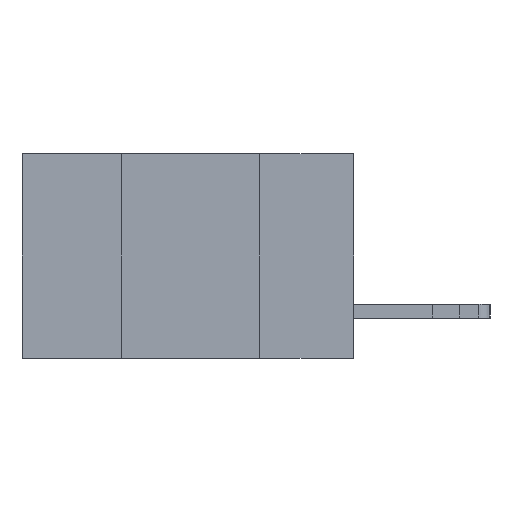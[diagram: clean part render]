
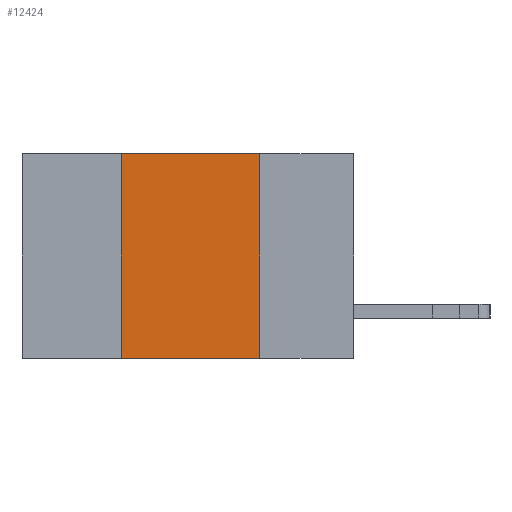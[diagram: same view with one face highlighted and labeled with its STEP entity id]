
A CAD part, left-side view. The second image highlights one B-rep face of the part: STEP entity #12424.
In plain terms, the highlighted planar face has unit normal (-1, 0, 0).
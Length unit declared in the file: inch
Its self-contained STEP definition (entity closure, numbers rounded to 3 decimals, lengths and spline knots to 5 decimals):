
#38 = ORIENTED_EDGE ( 'NONE', *, *, #11321, .T. ) ;
#1135 = PLANE ( 'NONE',  #7388 ) ;
#2249 = LINE ( 'NONE', #14327, #2546 ) ;
#2467 = VERTEX_POINT ( 'NONE', #12684 ) ;
#2546 = VECTOR ( 'NONE', #13043, 39.37008 ) ;
#2879 = DIRECTION ( 'NONE',  ( 0., 0., -1. ) ) ;
#2998 = EDGE_LOOP ( 'NONE', ( #4206, #7370, #8104, #38 ) ) ;
#3791 = CARTESIAN_POINT ( 'NONE',  ( 0., 0.17, 0. ) ) ;
#4206 = ORIENTED_EDGE ( 'NONE', *, *, #8826, .F. ) ;
#5432 = VECTOR ( 'NONE', #2879, 39.37008 ) ;
#5677 = VERTEX_POINT ( 'NONE', #6465 ) ;
#5744 = VERTEX_POINT ( 'NONE', #3791 ) ;
#6008 = CARTESIAN_POINT ( 'NONE',  ( 0., 0.6, 0. ) ) ;
#6465 = CARTESIAN_POINT ( 'NONE',  ( 0., 0.42, -0.37 ) ) ;
#7208 = VECTOR ( 'NONE', #13847, 39.37008 ) ;
#7370 = ORIENTED_EDGE ( 'NONE', *, *, #10621, .F. ) ;
#7388 = AXIS2_PLACEMENT_3D ( 'NONE', #16301, #15054, #8545 ) ;
#7578 = FACE_OUTER_BOUND ( 'NONE', #2998, .T. ) ;
#8104 = ORIENTED_EDGE ( 'NONE', *, *, #16740, .F. ) ;
#8545 = DIRECTION ( 'NONE',  ( 0., 0., -1. ) ) ;
#8826 = EDGE_CURVE ( 'NONE', #5744, #14418, #10849, .T. ) ;
#10621 = EDGE_CURVE ( 'NONE', #2467, #5744, #14060, .T. ) ;
#10849 = LINE ( 'NONE', #16007, #5432 ) ;
#11321 = EDGE_CURVE ( 'NONE', #5677, #14418, #12236, .T. ) ;
#12236 = LINE ( 'NONE', #12313, #7208 ) ;
#12313 = CARTESIAN_POINT ( 'NONE',  ( 0., 0.6, -0.37 ) ) ;
#12424 = ADVANCED_FACE ( 'NONE', ( #7578 ), #1135, .F. ) ;
#12659 = CARTESIAN_POINT ( 'NONE',  ( 0., 0.17, -0.37 ) ) ;
#12684 = CARTESIAN_POINT ( 'NONE',  ( 0., 0.42, 0. ) ) ;
#13043 = DIRECTION ( 'NONE',  ( 0., 0., 1. ) ) ;
#13847 = DIRECTION ( 'NONE',  ( 0., -1., 0. ) ) ;
#14060 = LINE ( 'NONE', #6008, #15450 ) ;
#14327 = CARTESIAN_POINT ( 'NONE',  ( 0., 0.42, 0. ) ) ;
#14418 = VERTEX_POINT ( 'NONE', #12659 ) ;
#15054 = DIRECTION ( 'NONE',  ( 1., 0., 0. ) ) ;
#15238 = DIRECTION ( 'NONE',  ( 0., -1., 0. ) ) ;
#15450 = VECTOR ( 'NONE', #15238, 39.37008 ) ;
#16007 = CARTESIAN_POINT ( 'NONE',  ( 0., 0.17, 0. ) ) ;
#16301 = CARTESIAN_POINT ( 'NONE',  ( 0., 0.6, 0. ) ) ;
#16740 = EDGE_CURVE ( 'NONE', #5677, #2467, #2249, .T. ) ;
